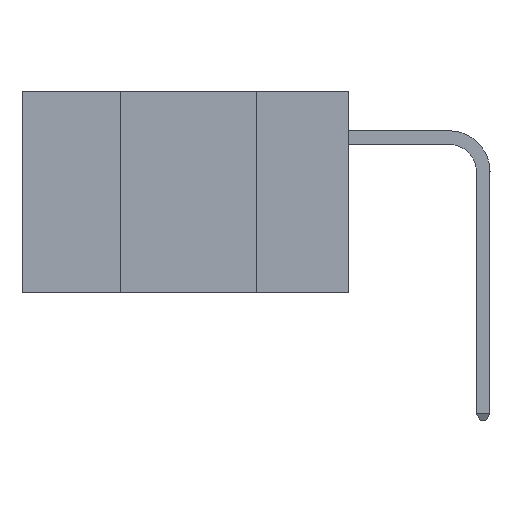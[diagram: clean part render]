
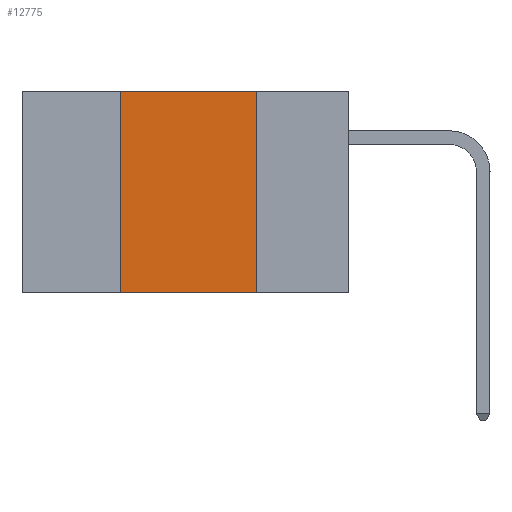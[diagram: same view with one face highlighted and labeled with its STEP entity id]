
A CAD part, left-side view. The second image highlights one B-rep face of the part: STEP entity #12775.
In plain terms, the highlighted planar face has unit normal (-1, 0, 0).
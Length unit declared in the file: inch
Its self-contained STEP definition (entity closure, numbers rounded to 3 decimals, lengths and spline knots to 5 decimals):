
#970 = VERTEX_POINT ( 'NONE', #46498 ) ;
#2169 = EDGE_LOOP ( 'NONE', ( #21635, #44059, #48088, #49545 ) ) ;
#2283 = AXIS2_PLACEMENT_3D ( 'NONE', #30931, #15285, #42862 ) ;
#2468 = LINE ( 'NONE', #19262, #18694 ) ;
#3238 = VECTOR ( 'NONE', #43058, 39.37008 ) ;
#10189 = VECTOR ( 'NONE', #25948, 39.37008 ) ;
#10981 = CARTESIAN_POINT ( 'NONE',  ( 0., 0.6, -0.37 ) ) ;
#11417 = LINE ( 'NONE', #44553, #10189 ) ;
#12775 = ADVANCED_FACE ( 'NONE', ( #27689 ), #46347, .F. ) ;
#13623 = VERTEX_POINT ( 'NONE', #28487 ) ;
#15245 = VERTEX_POINT ( 'NONE', #35592 ) ;
#15285 = DIRECTION ( 'NONE',  ( 1., 0., 0. ) ) ;
#18694 = VECTOR ( 'NONE', #19419, 39.37008 ) ;
#19262 = CARTESIAN_POINT ( 'NONE',  ( 0., 0.17, 0. ) ) ;
#19419 = DIRECTION ( 'NONE',  ( 0., 0., -1. ) ) ;
#19469 = VERTEX_POINT ( 'NONE', #46417 ) ;
#21635 = ORIENTED_EDGE ( 'NONE', *, *, #31358, .F. ) ;
#22250 = LINE ( 'NONE', #10981, #24755 ) ;
#24755 = VECTOR ( 'NONE', #26266, 39.37008 ) ;
#25948 = DIRECTION ( 'NONE',  ( 0., 0., 1. ) ) ;
#26266 = DIRECTION ( 'NONE',  ( 0., -1., 0. ) ) ;
#27689 = FACE_OUTER_BOUND ( 'NONE', #2169, .T. ) ;
#28487 = CARTESIAN_POINT ( 'NONE',  ( 0., 0.42, -0.37 ) ) ;
#29975 = LINE ( 'NONE', #39417, #3238 ) ;
#30931 = CARTESIAN_POINT ( 'NONE',  ( 0., 0.6, 0. ) ) ;
#31358 = EDGE_CURVE ( 'NONE', #15245, #970, #2468, .T. ) ;
#35592 = CARTESIAN_POINT ( 'NONE',  ( 0., 0.17, 0. ) ) ;
#39417 = CARTESIAN_POINT ( 'NONE',  ( 0., 0.6, 0. ) ) ;
#42862 = DIRECTION ( 'NONE',  ( 0., 0., -1. ) ) ;
#43058 = DIRECTION ( 'NONE',  ( 0., -1., 0. ) ) ;
#44059 = ORIENTED_EDGE ( 'NONE', *, *, #49122, .F. ) ;
#44553 = CARTESIAN_POINT ( 'NONE',  ( 0., 0.42, 0. ) ) ;
#45450 = EDGE_CURVE ( 'NONE', #13623, #970, #22250, .T. ) ;
#46347 = PLANE ( 'NONE',  #2283 ) ;
#46417 = CARTESIAN_POINT ( 'NONE',  ( 0., 0.42, 0. ) ) ;
#46498 = CARTESIAN_POINT ( 'NONE',  ( 0., 0.17, -0.37 ) ) ;
#48088 = ORIENTED_EDGE ( 'NONE', *, *, #48177, .F. ) ;
#48177 = EDGE_CURVE ( 'NONE', #13623, #19469, #11417, .T. ) ;
#49122 = EDGE_CURVE ( 'NONE', #19469, #15245, #29975, .T. ) ;
#49545 = ORIENTED_EDGE ( 'NONE', *, *, #45450, .T. ) ;
